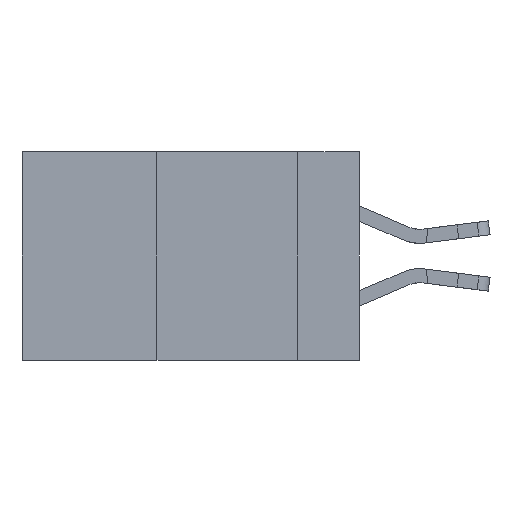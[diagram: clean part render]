
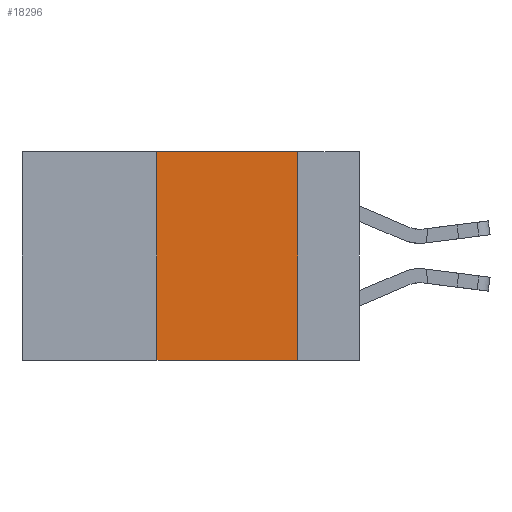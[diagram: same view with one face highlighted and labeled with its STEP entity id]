
A CAD part, left-side view. The second image highlights one B-rep face of the part: STEP entity #18296.
In plain terms, the highlighted planar face has unit normal (-1, 0, 0).
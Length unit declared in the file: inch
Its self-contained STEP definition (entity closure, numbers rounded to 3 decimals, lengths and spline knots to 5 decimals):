
#73 = EDGE_CURVE ( 'NONE', #22812, #28049, #8207, .T. ) ;
#455 = CARTESIAN_POINT ( 'NONE',  ( 0., 0.6, -0.37 ) ) ;
#1941 = VECTOR ( 'NONE', #32227, 39.37008 ) ;
#2459 = DIRECTION ( 'NONE',  ( 0., -1., 0. ) ) ;
#4381 = LINE ( 'NONE', #455, #1941 ) ;
#4431 = ORIENTED_EDGE ( 'NONE', *, *, #73, .F. ) ;
#4556 = ORIENTED_EDGE ( 'NONE', *, *, #27489, .F. ) ;
#5125 = FACE_OUTER_BOUND ( 'NONE', #22640, .T. ) ;
#5566 = CARTESIAN_POINT ( 'NONE',  ( 0., 0.11, 0. ) ) ;
#5832 = CARTESIAN_POINT ( 'NONE',  ( 0., 0.36, 0. ) ) ;
#5911 = LINE ( 'NONE', #25260, #24497 ) ;
#7165 = CARTESIAN_POINT ( 'NONE',  ( 0., 0.6, 0. ) ) ;
#8046 = VECTOR ( 'NONE', #21118, 39.37008 ) ;
#8207 = LINE ( 'NONE', #24109, #18919 ) ;
#15126 = VERTEX_POINT ( 'NONE', #19004 ) ;
#16285 = DIRECTION ( 'NONE',  ( 0., 0., -1. ) ) ;
#17544 = DIRECTION ( 'NONE',  ( 1., 0., 0. ) ) ;
#18296 = ADVANCED_FACE ( 'NONE', ( #5125 ), #33081, .F. ) ;
#18919 = VECTOR ( 'NONE', #16285, 39.37008 ) ;
#19004 = CARTESIAN_POINT ( 'NONE',  ( 0., 0.36, -0.37 ) ) ;
#21118 = DIRECTION ( 'NONE',  ( 0., 0., 1. ) ) ;
#21313 = VERTEX_POINT ( 'NONE', #5832 ) ;
#22403 = ORIENTED_EDGE ( 'NONE', *, *, #22824, .T. ) ;
#22640 = EDGE_LOOP ( 'NONE', ( #4431, #4556, #32325, #22403 ) ) ;
#22812 = VERTEX_POINT ( 'NONE', #5566 ) ;
#22824 = EDGE_CURVE ( 'NONE', #15126, #28049, #4381, .T. ) ;
#23276 = CARTESIAN_POINT ( 'NONE',  ( 0., 0.11, -0.37 ) ) ;
#23912 = EDGE_CURVE ( 'NONE', #15126, #21313, #30278, .T. ) ;
#24109 = CARTESIAN_POINT ( 'NONE',  ( 0., 0.11, 0. ) ) ;
#24497 = VECTOR ( 'NONE', #2459, 39.37008 ) ;
#25260 = CARTESIAN_POINT ( 'NONE',  ( 0., 0.6, 0. ) ) ;
#25369 = DIRECTION ( 'NONE',  ( 0., 0., -1. ) ) ;
#26865 = AXIS2_PLACEMENT_3D ( 'NONE', #7165, #17544, #25369 ) ;
#27489 = EDGE_CURVE ( 'NONE', #21313, #22812, #5911, .T. ) ;
#28049 = VERTEX_POINT ( 'NONE', #23276 ) ;
#30278 = LINE ( 'NONE', #31823, #8046 ) ;
#31823 = CARTESIAN_POINT ( 'NONE',  ( 0., 0.36, 0. ) ) ;
#32227 = DIRECTION ( 'NONE',  ( 0., -1., 0. ) ) ;
#32325 = ORIENTED_EDGE ( 'NONE', *, *, #23912, .F. ) ;
#33081 = PLANE ( 'NONE',  #26865 ) ;
